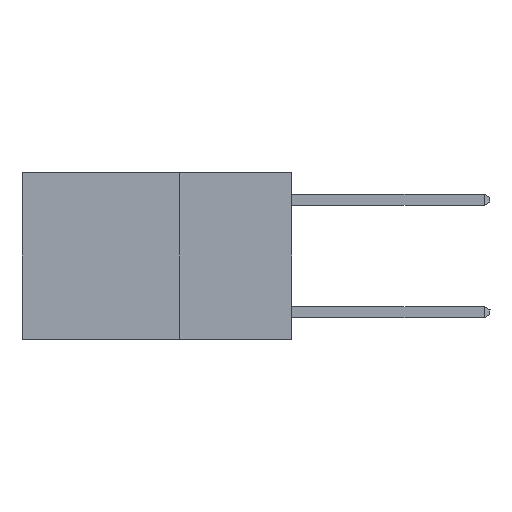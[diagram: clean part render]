
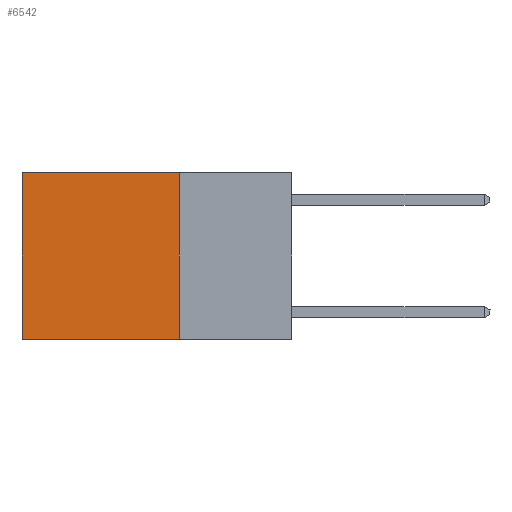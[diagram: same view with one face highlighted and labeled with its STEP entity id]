
A CAD part, left-side view. The second image highlights one B-rep face of the part: STEP entity #6542.
In plain terms, the highlighted planar face has unit normal (-1, 0, 0).
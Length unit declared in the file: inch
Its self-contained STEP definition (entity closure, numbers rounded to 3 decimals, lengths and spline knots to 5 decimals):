
#247 = LINE ( 'NONE', #7172, #15014 ) ;
#1744 = VERTEX_POINT ( 'NONE', #15744 ) ;
#1974 = DIRECTION ( 'NONE',  ( 0., 0., -1. ) ) ;
#2084 = LINE ( 'NONE', #10049, #7112 ) ;
#2109 = EDGE_CURVE ( 'NONE', #1744, #2124, #247, .T. ) ;
#2124 = VERTEX_POINT ( 'NONE', #11306 ) ;
#2965 = ORIENTED_EDGE ( 'NONE', *, *, #2109, .T. ) ;
#3632 = CARTESIAN_POINT ( 'NONE',  ( 0.2625, 0.25, -0.37 ) ) ;
#4054 = EDGE_CURVE ( 'NONE', #1744, #13942, #5752, .T. ) ;
#5752 = LINE ( 'NONE', #12033, #12495 ) ;
#6194 = DIRECTION ( 'NONE',  ( 0., 1., 0. ) ) ;
#6542 = ADVANCED_FACE ( 'NONE', ( #7295 ), #8701, .F. ) ;
#6569 = CARTESIAN_POINT ( 'NONE',  ( 0.2625, 0.6, -0.37 ) ) ;
#7112 = VECTOR ( 'NONE', #15594, 39.37008 ) ;
#7172 = CARTESIAN_POINT ( 'NONE',  ( 0.2625, 0.25, 0. ) ) ;
#7295 = FACE_OUTER_BOUND ( 'NONE', #10960, .T. ) ;
#8701 = PLANE ( 'NONE',  #15729 ) ;
#8776 = ORIENTED_EDGE ( 'NONE', *, *, #12290, .T. ) ;
#10049 = CARTESIAN_POINT ( 'NONE',  ( 0.2625, 0.6, 0. ) ) ;
#10960 = EDGE_LOOP ( 'NONE', ( #8776, #13665, #14596, #2965 ) ) ;
#11306 = CARTESIAN_POINT ( 'NONE',  ( 0.2625, 0.6, 0. ) ) ;
#11622 = VERTEX_POINT ( 'NONE', #6569 ) ;
#12033 = CARTESIAN_POINT ( 'NONE',  ( 0.2625, 0.25, 0. ) ) ;
#12290 = EDGE_CURVE ( 'NONE', #2124, #11622, #2084, .T. ) ;
#12495 = VECTOR ( 'NONE', #16545, 39.37008 ) ;
#12559 = VECTOR ( 'NONE', #6194, 39.37008 ) ;
#12578 = CARTESIAN_POINT ( 'NONE',  ( 0.2625, 0.25, 0. ) ) ;
#13665 = ORIENTED_EDGE ( 'NONE', *, *, #16872, .F. ) ;
#13942 = VERTEX_POINT ( 'NONE', #17420 ) ;
#14119 = DIRECTION ( 'NONE',  ( 1., 0., 0. ) ) ;
#14596 = ORIENTED_EDGE ( 'NONE', *, *, #4054, .F. ) ;
#15014 = VECTOR ( 'NONE', #15518, 39.37008 ) ;
#15518 = DIRECTION ( 'NONE',  ( 0., 1., 0. ) ) ;
#15594 = DIRECTION ( 'NONE',  ( 0., 0., -1. ) ) ;
#15729 = AXIS2_PLACEMENT_3D ( 'NONE', #12578, #14119, #1974 ) ;
#15744 = CARTESIAN_POINT ( 'NONE',  ( 0.2625, 0.25, 0. ) ) ;
#15852 = LINE ( 'NONE', #3632, #12559 ) ;
#16545 = DIRECTION ( 'NONE',  ( 0., 0., -1. ) ) ;
#16872 = EDGE_CURVE ( 'NONE', #13942, #11622, #15852, .T. ) ;
#17420 = CARTESIAN_POINT ( 'NONE',  ( 0.2625, 0.25, -0.37 ) ) ;
